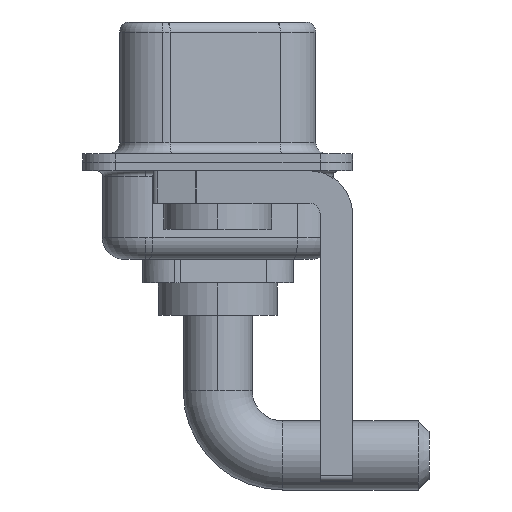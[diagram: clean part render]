
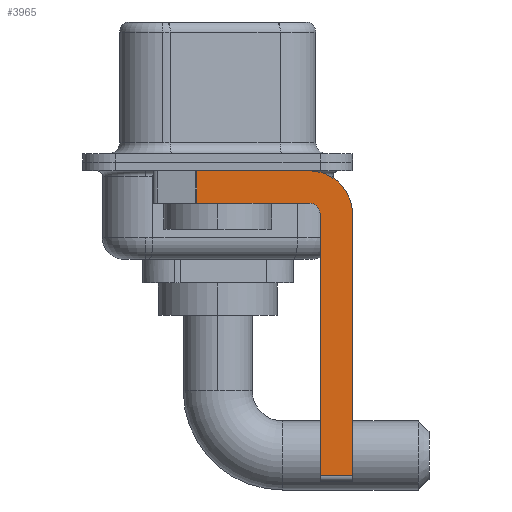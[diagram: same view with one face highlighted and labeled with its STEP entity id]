
A CAD part, left-side view. The second image highlights one B-rep face of the part: STEP entity #3965.
In plain terms, the highlighted planar face has unit normal (-1, 0, 0).
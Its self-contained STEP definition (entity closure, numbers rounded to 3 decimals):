
#125 = LINE ( 'NONE', #13471, #4815 ) ;
#372 = CARTESIAN_POINT ( 'NONE',  ( -2.9, -4.25, -2.4 ) ) ;
#477 = EDGE_LOOP ( 'NONE', ( #14954, #7216, #6326, #2840, #3455, #16551, #2360, #3713 ) ) ;
#1262 = LINE ( 'NONE', #6840, #13615 ) ;
#1689 = PLANE ( 'NONE',  #16833 ) ;
#1796 = VECTOR ( 'NONE', #14208, 1000. ) ;
#1897 = EDGE_CURVE ( 'NONE', #9575, #2319, #15006, .T. ) ;
#2180 = EDGE_CURVE ( 'NONE', #13510, #11221, #9557, .T. ) ;
#2319 = VERTEX_POINT ( 'NONE', #12233 ) ;
#2360 = ORIENTED_EDGE ( 'NONE', *, *, #7948, .F. ) ;
#2493 = VERTEX_POINT ( 'NONE', #6446 ) ;
#2840 = ORIENTED_EDGE ( 'NONE', *, *, #5703, .F. ) ;
#2950 = VERTEX_POINT ( 'NONE', #9085 ) ;
#3455 = ORIENTED_EDGE ( 'NONE', *, *, #1897, .F. ) ;
#3713 = ORIENTED_EDGE ( 'NONE', *, *, #10242, .F. ) ;
#3965 = ADVANCED_FACE ( 'NONE', ( #10750 ), #1689, .F. ) ;
#4230 = DIRECTION ( 'NONE',  ( 1., 0., 0. ) ) ;
#4815 = VECTOR ( 'NONE', #6585, 1000. ) ;
#5703 = EDGE_CURVE ( 'NONE', #2319, #2950, #10409, .T. ) ;
#6138 = CARTESIAN_POINT ( 'NONE',  ( -2.9, 0.978, -0.4 ) ) ;
#6326 = ORIENTED_EDGE ( 'NONE', *, *, #14558, .F. ) ;
#6446 = CARTESIAN_POINT ( 'NONE',  ( -2.9, -6.25, -14.55 ) ) ;
#6585 = DIRECTION ( 'NONE',  ( 0., 1., 0. ) ) ;
#6840 = CARTESIAN_POINT ( 'NONE',  ( -2.9, 0.978, -1.9 ) ) ;
#6933 = DIRECTION ( 'NONE',  ( 0., 0., -1. ) ) ;
#7216 = ORIENTED_EDGE ( 'NONE', *, *, #9826, .T. ) ;
#7742 = LINE ( 'NONE', #7821, #1796 ) ;
#7821 = CARTESIAN_POINT ( 'NONE',  ( -2.9, -4.25, -14.55 ) ) ;
#7948 = EDGE_CURVE ( 'NONE', #11290, #2493, #12129, .T. ) ;
#8114 = CARTESIAN_POINT ( 'NONE',  ( -2.9, -4.25, -2.4 ) ) ;
#8571 = CARTESIAN_POINT ( 'NONE',  ( -2.9, -4.25, -0.4 ) ) ;
#8834 = CARTESIAN_POINT ( 'NONE',  ( -2.9, -6.25, -2.4 ) ) ;
#9085 = CARTESIAN_POINT ( 'NONE',  ( -2.9, -4.25, -1.9 ) ) ;
#9510 = DIRECTION ( 'NONE',  ( 0., 0., -1. ) ) ;
#9557 = LINE ( 'NONE', #14828, #11065 ) ;
#9575 = VERTEX_POINT ( 'NONE', #11697 ) ;
#9826 = EDGE_CURVE ( 'NONE', #13510, #14217, #1262, .T. ) ;
#10242 = EDGE_CURVE ( 'NONE', #11221, #11290, #11113, .T. ) ;
#10409 = CIRCLE ( 'NONE', #13423, 0.5 ) ;
#10750 = FACE_OUTER_BOUND ( 'NONE', #477, .T. ) ;
#11044 = DIRECTION ( 'NONE',  ( 0., 0., 1. ) ) ;
#11065 = VECTOR ( 'NONE', #13193, 1000. ) ;
#11085 = CARTESIAN_POINT ( 'NONE',  ( -2.9, 0.978, -1.9 ) ) ;
#11113 = CIRCLE ( 'NONE', #14695, 2. ) ;
#11221 = VERTEX_POINT ( 'NONE', #8571 ) ;
#11290 = VERTEX_POINT ( 'NONE', #8834 ) ;
#11697 = CARTESIAN_POINT ( 'NONE',  ( -2.9, -4.75, -14.55 ) ) ;
#12129 = LINE ( 'NONE', #13760, #15618 ) ;
#12204 = DIRECTION ( 'NONE',  ( 1., 0., 0. ) ) ;
#12233 = CARTESIAN_POINT ( 'NONE',  ( -2.9, -4.75, -2.4 ) ) ;
#12379 = DIRECTION ( 'NONE',  ( 0., 0., -1. ) ) ;
#13193 = DIRECTION ( 'NONE',  ( 0., -1., 0. ) ) ;
#13423 = AXIS2_PLACEMENT_3D ( 'NONE', #372, #13555, #13647 ) ;
#13471 = CARTESIAN_POINT ( 'NONE',  ( -2.9, -4.25, -1.9 ) ) ;
#13510 = VERTEX_POINT ( 'NONE', #6138 ) ;
#13555 = DIRECTION ( 'NONE',  ( -1., 0., 0. ) ) ;
#13615 = VECTOR ( 'NONE', #9510, 1000. ) ;
#13647 = DIRECTION ( 'NONE',  ( 0., 0., 1. ) ) ;
#13760 = CARTESIAN_POINT ( 'NONE',  ( -2.9, -6.25, -2.4 ) ) ;
#13901 = EDGE_CURVE ( 'NONE', #9575, #2493, #7742, .T. ) ;
#14208 = DIRECTION ( 'NONE',  ( 0., -1., 0. ) ) ;
#14217 = VERTEX_POINT ( 'NONE', #11085 ) ;
#14558 = EDGE_CURVE ( 'NONE', #2950, #14217, #125, .T. ) ;
#14695 = AXIS2_PLACEMENT_3D ( 'NONE', #8114, #4230, #14930 ) ;
#14828 = CARTESIAN_POINT ( 'NONE',  ( -2.9, 3., -0.4 ) ) ;
#14930 = DIRECTION ( 'NONE',  ( 0., 0., -1. ) ) ;
#14954 = ORIENTED_EDGE ( 'NONE', *, *, #2180, .F. ) ;
#14961 = CARTESIAN_POINT ( 'NONE',  ( -2.9, -4.25, -2.4 ) ) ;
#15006 = LINE ( 'NONE', #16478, #16318 ) ;
#15618 = VECTOR ( 'NONE', #6933, 1000. ) ;
#16318 = VECTOR ( 'NONE', #11044, 1000. ) ;
#16478 = CARTESIAN_POINT ( 'NONE',  ( -2.9, -4.75, -14.8 ) ) ;
#16551 = ORIENTED_EDGE ( 'NONE', *, *, #13901, .T. ) ;
#16833 = AXIS2_PLACEMENT_3D ( 'NONE', #14961, #12204, #12379 ) ;
